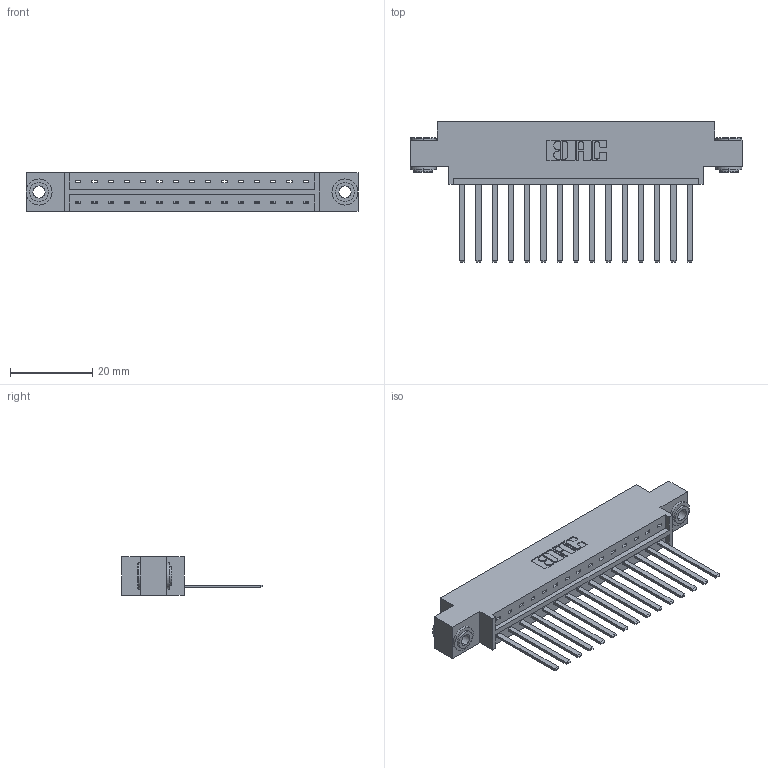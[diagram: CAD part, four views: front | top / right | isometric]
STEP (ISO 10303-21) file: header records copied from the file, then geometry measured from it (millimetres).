
FILE_DESCRIPTION (( 'STEP AP203' ), '1' );
FILE_NAME ('333-015-544-603.STEP', '2018-08-01T04:00:12', ( '' ), ( '' ), 'SwSTEP 2.0', 'SolidWorks 2016', '' );
FILE_SCHEMA (( 'CONFIG_CONTROL_DESIGN' ));
Length unit declared in the file: inch
Products named in the file (4): 345-250-002_345-250-002-102; 333-015-544-603; 333 Part_Offset - .156 Dia - TH; 345-292-001_345-293-144
Assembly tree (18 placements, depth 2):
  333-015-544-603
    333 Part_Offset - .156 Dia - TH
    345-292-001_345-293-144  x15
    345-250-002_345-250-002-102  x2
Bounding box: 80.98 x 34.3 x 9.4 mm (x, y, z)
Volume: 7881.5 mm3; surface area: 9341.4 mm2
Topology: 18 solids, 18 shells, 936 faces, 2769 edges, 1822 vertices
Faces by surface type: plane 654, cylinder 274, cone 8
Entity records: 13260 total; most frequent: CARTESIAN_POINT 2270, ORIENTED_EDGE 2214, DIRECTION 1999, EDGE_CURVE 1107, VECTOR 959, LINE 959, VERTEX_POINT 734, AXIS2_PLACEMENT_3D 520
